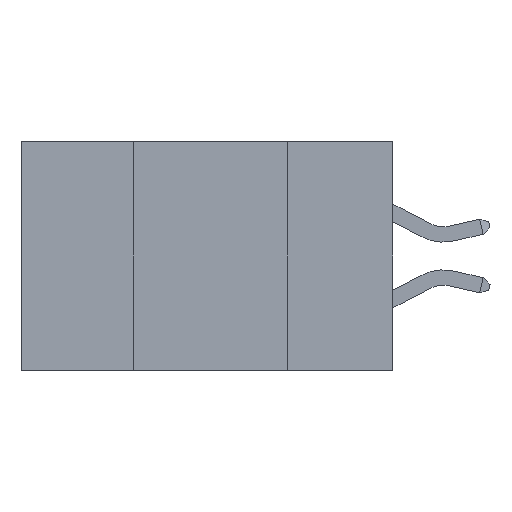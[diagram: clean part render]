
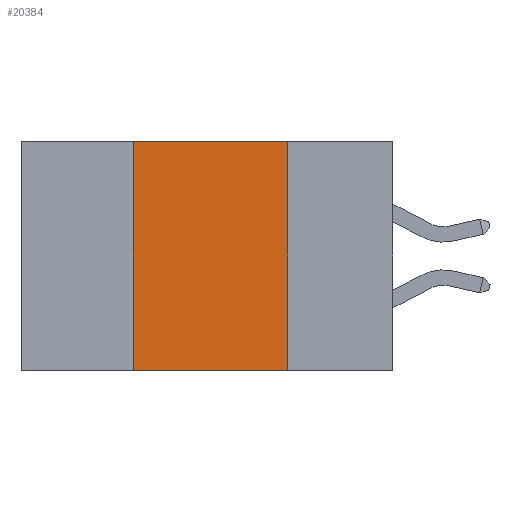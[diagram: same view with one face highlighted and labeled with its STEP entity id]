
A CAD part, left-side view. The second image highlights one B-rep face of the part: STEP entity #20384.
In plain terms, the highlighted planar face has unit normal (-1, 0, 0).
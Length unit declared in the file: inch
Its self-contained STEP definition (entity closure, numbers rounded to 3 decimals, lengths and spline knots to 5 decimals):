
#2967 = EDGE_CURVE ( 'NONE', #19530, #17727, #15817, .T. ) ;
#3126 = VECTOR ( 'NONE', #13141, 39.37008 ) ;
#4188 = CARTESIAN_POINT ( 'NONE',  ( 0., 0.6, 0. ) ) ;
#4678 = CARTESIAN_POINT ( 'NONE',  ( 0., 0.6, 0. ) ) ;
#5318 = CARTESIAN_POINT ( 'NONE',  ( 0., 0.6, -0.37 ) ) ;
#5628 = FACE_OUTER_BOUND ( 'NONE', #17869, .T. ) ;
#5645 = CARTESIAN_POINT ( 'NONE',  ( 0., 0.17, 0. ) ) ;
#5998 = LINE ( 'NONE', #5318, #14472 ) ;
#6608 = VECTOR ( 'NONE', #8738, 39.37008 ) ;
#7582 = CARTESIAN_POINT ( 'NONE',  ( 0., 0.17, 0. ) ) ;
#8738 = DIRECTION ( 'NONE',  ( 0., 0., 1. ) ) ;
#9091 = CARTESIAN_POINT ( 'NONE',  ( 0., 0.42, -0.37 ) ) ;
#9669 = CARTESIAN_POINT ( 'NONE',  ( 0., 0.42, 0. ) ) ;
#10435 = VECTOR ( 'NONE', #12900, 39.37008 ) ;
#10868 = AXIS2_PLACEMENT_3D ( 'NONE', #4678, #22694, #11910 ) ;
#11338 = ORIENTED_EDGE ( 'NONE', *, *, #13437, .F. ) ;
#11910 = DIRECTION ( 'NONE',  ( 0., 0., -1. ) ) ;
#12900 = DIRECTION ( 'NONE',  ( 0., 0., -1. ) ) ;
#13141 = DIRECTION ( 'NONE',  ( 0., -1., 0. ) ) ;
#13437 = EDGE_CURVE ( 'NONE', #14676, #19530, #22284, .T. ) ;
#14118 = CARTESIAN_POINT ( 'NONE',  ( 0., 0.42, 0. ) ) ;
#14472 = VECTOR ( 'NONE', #19761, 39.37008 ) ;
#14676 = VERTEX_POINT ( 'NONE', #9669 ) ;
#15477 = PLANE ( 'NONE',  #10868 ) ;
#15669 = VERTEX_POINT ( 'NONE', #9091 ) ;
#15817 = LINE ( 'NONE', #5645, #10435 ) ;
#16722 = EDGE_CURVE ( 'NONE', #15669, #14676, #21596, .T. ) ;
#16926 = CARTESIAN_POINT ( 'NONE',  ( 0., 0.17, -0.37 ) ) ;
#17727 = VERTEX_POINT ( 'NONE', #16926 ) ;
#17869 = EDGE_LOOP ( 'NONE', ( #21772, #11338, #19552, #21229 ) ) ;
#18054 = EDGE_CURVE ( 'NONE', #15669, #17727, #5998, .T. ) ;
#19530 = VERTEX_POINT ( 'NONE', #7582 ) ;
#19552 = ORIENTED_EDGE ( 'NONE', *, *, #16722, .F. ) ;
#19761 = DIRECTION ( 'NONE',  ( 0., -1., 0. ) ) ;
#20384 = ADVANCED_FACE ( 'NONE', ( #5628 ), #15477, .F. ) ;
#21229 = ORIENTED_EDGE ( 'NONE', *, *, #18054, .T. ) ;
#21596 = LINE ( 'NONE', #14118, #6608 ) ;
#21772 = ORIENTED_EDGE ( 'NONE', *, *, #2967, .F. ) ;
#22284 = LINE ( 'NONE', #4188, #3126 ) ;
#22694 = DIRECTION ( 'NONE',  ( 1., 0., 0. ) ) ;
